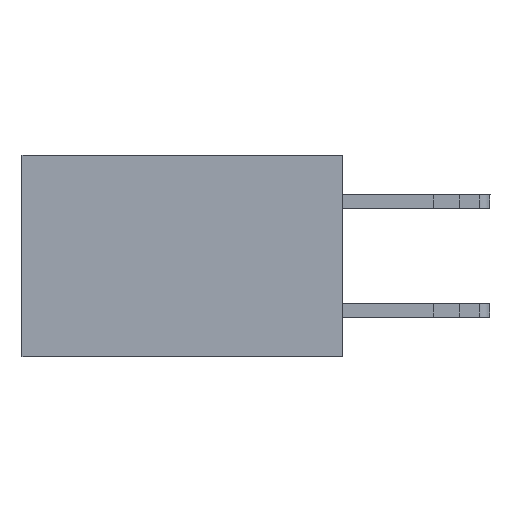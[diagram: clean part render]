
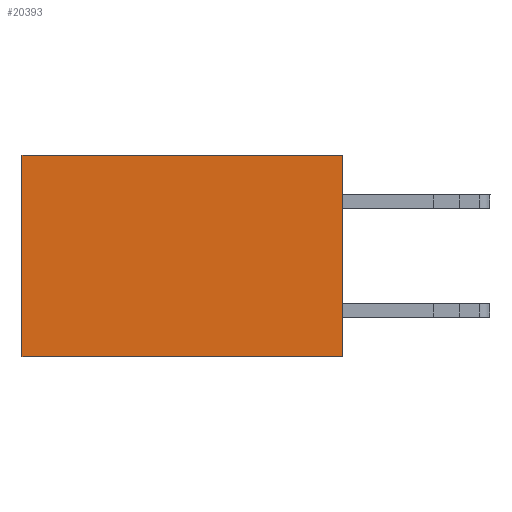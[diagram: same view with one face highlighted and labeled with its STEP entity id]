
A CAD part, left-side view. The second image highlights one B-rep face of the part: STEP entity #20393.
In plain terms, the highlighted planar face has unit normal (-1, 0, 0).
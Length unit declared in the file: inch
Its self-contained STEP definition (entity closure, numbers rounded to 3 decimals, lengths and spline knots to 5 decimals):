
#91 = AXIS2_PLACEMENT_3D ( 'NONE', #14940, #13180, #6093 ) ;
#743 = EDGE_CURVE ( 'NONE', #13094, #16936, #9349, .T. ) ;
#845 = ORIENTED_EDGE ( 'NONE', *, *, #25846, .F. ) ;
#1127 = LINE ( 'NONE', #7952, #3517 ) ;
#2396 = CARTESIAN_POINT ( 'NONE',  ( 0.277, 0.59, -0.37 ) ) ;
#3018 = ORIENTED_EDGE ( 'NONE', *, *, #743, .T. ) ;
#3399 = CARTESIAN_POINT ( 'NONE',  ( 0.277, 0., 0. ) ) ;
#3517 = VECTOR ( 'NONE', #21446, 39.37008 ) ;
#5798 = VECTOR ( 'NONE', #18897, 39.37008 ) ;
#5810 = EDGE_CURVE ( 'NONE', #7788, #13094, #6286, .T. ) ;
#5944 = CARTESIAN_POINT ( 'NONE',  ( 0.277, 0., -0.37 ) ) ;
#6093 = DIRECTION ( 'NONE',  ( 0., 0., -1. ) ) ;
#6286 = LINE ( 'NONE', #17007, #12698 ) ;
#6291 = CARTESIAN_POINT ( 'NONE',  ( 0.277, 0.59, -0.37 ) ) ;
#6423 = EDGE_LOOP ( 'NONE', ( #3018, #22263, #845, #22037 ) ) ;
#6624 = EDGE_CURVE ( 'NONE', #20219, #16936, #28317, .T. ) ;
#6647 = PLANE ( 'NONE',  #91 ) ;
#7788 = VERTEX_POINT ( 'NONE', #3399 ) ;
#7952 = CARTESIAN_POINT ( 'NONE',  ( 0.277, 0., -0.37 ) ) ;
#8796 = CARTESIAN_POINT ( 'NONE',  ( 0.277, 0.59, 0. ) ) ;
#9349 = LINE ( 'NONE', #2396, #22056 ) ;
#12698 = VECTOR ( 'NONE', #19612, 39.37008 ) ;
#13094 = VERTEX_POINT ( 'NONE', #8796 ) ;
#13180 = DIRECTION ( 'NONE',  ( 1., 0., 0. ) ) ;
#13317 = FACE_OUTER_BOUND ( 'NONE', #6423, .T. ) ;
#14848 = CARTESIAN_POINT ( 'NONE',  ( 0.277, 0., -0.37 ) ) ;
#14940 = CARTESIAN_POINT ( 'NONE',  ( 0.277, 0., -0.37 ) ) ;
#15727 = DIRECTION ( 'NONE',  ( 0., 0., -1. ) ) ;
#16936 = VERTEX_POINT ( 'NONE', #6291 ) ;
#17007 = CARTESIAN_POINT ( 'NONE',  ( 0.277, 0., 0. ) ) ;
#18897 = DIRECTION ( 'NONE',  ( 0., 1., 0. ) ) ;
#19612 = DIRECTION ( 'NONE',  ( 0., 1., 0. ) ) ;
#20219 = VERTEX_POINT ( 'NONE', #5944 ) ;
#20393 = ADVANCED_FACE ( 'NONE', ( #13317 ), #6647, .F. ) ;
#21446 = DIRECTION ( 'NONE',  ( 0., 0., -1. ) ) ;
#22037 = ORIENTED_EDGE ( 'NONE', *, *, #5810, .T. ) ;
#22056 = VECTOR ( 'NONE', #15727, 39.37008 ) ;
#22263 = ORIENTED_EDGE ( 'NONE', *, *, #6624, .F. ) ;
#25846 = EDGE_CURVE ( 'NONE', #7788, #20219, #1127, .T. ) ;
#28317 = LINE ( 'NONE', #14848, #5798 ) ;
